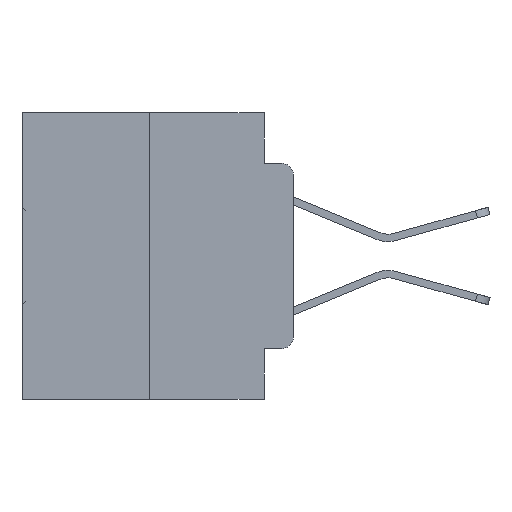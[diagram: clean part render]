
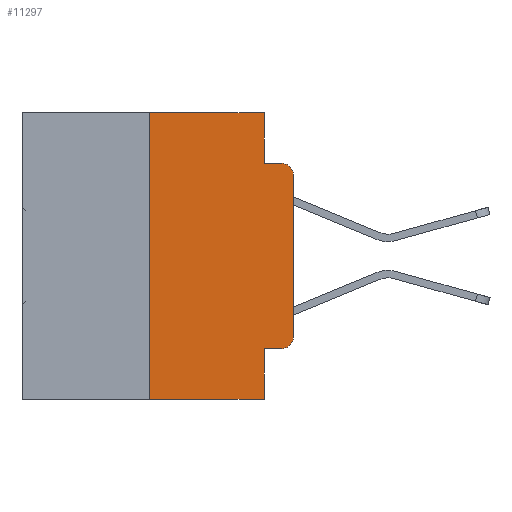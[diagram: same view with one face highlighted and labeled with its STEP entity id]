
A CAD part, left-side view. The second image highlights one B-rep face of the part: STEP entity #11297.
In plain terms, the highlighted planar face has unit normal (-1, 0, 0).
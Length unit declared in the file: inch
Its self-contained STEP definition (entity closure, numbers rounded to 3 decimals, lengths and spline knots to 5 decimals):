
#302 = DIRECTION ( 'NONE',  ( -1., 0., 0. ) ) ;
#361 = PLANE ( 'NONE',  #14105 ) ;
#1832 = EDGE_CURVE ( 'NONE', #31508, #29233, #28440, .T. ) ;
#3034 = VECTOR ( 'NONE', #4120, 39.37008 ) ;
#3745 = VECTOR ( 'NONE', #17222, 39.37008 ) ;
#3952 = DIRECTION ( 'NONE',  ( 0., -1., 0. ) ) ;
#4120 = DIRECTION ( 'NONE',  ( 0., 0., 1. ) ) ;
#5749 = ORIENTED_EDGE ( 'NONE', *, *, #12682, .T. ) ;
#5915 = DIRECTION ( 'NONE',  ( 0., 0., -1. ) ) ;
#6201 = LINE ( 'NONE', #6264, #7006 ) ;
#6264 = CARTESIAN_POINT ( 'NONE',  ( 0., 0.473, -0.5 ) ) ;
#7006 = VECTOR ( 'NONE', #24148, 39.37008 ) ;
#7079 = EDGE_CURVE ( 'NONE', #20912, #33186, #18273, .T. ) ;
#7255 = EDGE_LOOP ( 'NONE', ( #5749, #28667, #17162, #28207, #28958, #24762, #18702, #12947, #8277, #7651 ) ) ;
#7651 = ORIENTED_EDGE ( 'NONE', *, *, #7079, .T. ) ;
#7971 = LINE ( 'NONE', #11156, #21092 ) ;
#8277 = ORIENTED_EDGE ( 'NONE', *, *, #10899, .T. ) ;
#9403 = DIRECTION ( 'NONE',  ( 0., 0., -1. ) ) ;
#9429 = VECTOR ( 'NONE', #13624, 39.37008 ) ;
#9507 = CARTESIAN_POINT ( 'NONE',  ( 0., 0.02, -0.3915 ) ) ;
#10441 = CARTESIAN_POINT ( 'NONE',  ( 0., 0.051, 0. ) ) ;
#10899 = EDGE_CURVE ( 'NONE', #14200, #20912, #20010, .T. ) ;
#11002 = VERTEX_POINT ( 'NONE', #27409 ) ;
#11156 = CARTESIAN_POINT ( 'NONE',  ( 0., 0., 0. ) ) ;
#11297 = ADVANCED_FACE ( 'NONE', ( #21189 ), #361, .F. ) ;
#11696 = CARTESIAN_POINT ( 'NONE',  ( 0., 0.473, 0. ) ) ;
#12386 = VERTEX_POINT ( 'NONE', #24141 ) ;
#12682 = EDGE_CURVE ( 'NONE', #33186, #31508, #7971, .T. ) ;
#12947 = ORIENTED_EDGE ( 'NONE', *, *, #17543, .F. ) ;
#13279 = CARTESIAN_POINT ( 'NONE',  ( 0., 0.02, -0.1085 ) ) ;
#13501 = DIRECTION ( 'NONE',  ( 0., -1., 0. ) ) ;
#13624 = DIRECTION ( 'NONE',  ( 0., 0., -1. ) ) ;
#13856 = CARTESIAN_POINT ( 'NONE',  ( 0., 0., -0.1085 ) ) ;
#14105 = AXIS2_PLACEMENT_3D ( 'NONE', #24378, #16372, #5915 ) ;
#14200 = VERTEX_POINT ( 'NONE', #19577 ) ;
#14707 = EDGE_CURVE ( 'NONE', #12386, #29233, #19515, .T. ) ;
#16372 = DIRECTION ( 'NONE',  ( 1., 0., 0. ) ) ;
#16725 = EDGE_CURVE ( 'NONE', #23907, #30008, #27983, .T. ) ;
#17162 = ORIENTED_EDGE ( 'NONE', *, *, #14707, .F. ) ;
#17222 = DIRECTION ( 'NONE',  ( 0., -1., 0. ) ) ;
#17543 = EDGE_CURVE ( 'NONE', #14200, #18898, #30412, .T. ) ;
#18273 = CIRCLE ( 'NONE', #23080, 0.02 ) ;
#18702 = ORIENTED_EDGE ( 'NONE', *, *, #27818, .T. ) ;
#18712 = DIRECTION ( 'NONE',  ( 0., 0., -1. ) ) ;
#18898 = VERTEX_POINT ( 'NONE', #22165 ) ;
#18912 = DIRECTION ( 'NONE',  ( 0., 0., 1. ) ) ;
#19515 = LINE ( 'NONE', #32539, #25696 ) ;
#19577 = CARTESIAN_POINT ( 'NONE',  ( 0., 0.051, -0.4115 ) ) ;
#19688 = DIRECTION ( 'NONE',  ( 0., 0., -1. ) ) ;
#20010 = LINE ( 'NONE', #32227, #22914 ) ;
#20912 = VERTEX_POINT ( 'NONE', #33332 ) ;
#20940 = AXIS2_PLACEMENT_3D ( 'NONE', #13279, #302, #18712 ) ;
#21092 = VECTOR ( 'NONE', #18912, 39.37008 ) ;
#21101 = LINE ( 'NONE', #29957, #3034 ) ;
#21189 = FACE_OUTER_BOUND ( 'NONE', #7255, .T. ) ;
#21349 = LINE ( 'NONE', #10441, #9429 ) ;
#21358 = EDGE_CURVE ( 'NONE', #11002, #23907, #21101, .T. ) ;
#22165 = CARTESIAN_POINT ( 'NONE',  ( 0., 0.051, -0.5 ) ) ;
#22914 = VECTOR ( 'NONE', #13501, 39.37008 ) ;
#23080 = AXIS2_PLACEMENT_3D ( 'NONE', #9507, #30433, #9403 ) ;
#23406 = VECTOR ( 'NONE', #19688, 39.37008 ) ;
#23907 = VERTEX_POINT ( 'NONE', #26895 ) ;
#24141 = CARTESIAN_POINT ( 'NONE',  ( 0., 0.051, -0.0885 ) ) ;
#24148 = DIRECTION ( 'NONE',  ( 0., -1., 0. ) ) ;
#24378 = CARTESIAN_POINT ( 'NONE',  ( 0., 0.473, 0. ) ) ;
#24402 = EDGE_CURVE ( 'NONE', #30008, #12386, #21349, .T. ) ;
#24762 = ORIENTED_EDGE ( 'NONE', *, *, #21358, .F. ) ;
#25696 = VECTOR ( 'NONE', #3952, 39.37008 ) ;
#26895 = CARTESIAN_POINT ( 'NONE',  ( 0., 0.25, 0. ) ) ;
#27409 = CARTESIAN_POINT ( 'NONE',  ( 0., 0.25, -0.5 ) ) ;
#27818 = EDGE_CURVE ( 'NONE', #11002, #18898, #6201, .T. ) ;
#27983 = LINE ( 'NONE', #11696, #3745 ) ;
#28150 = CARTESIAN_POINT ( 'NONE',  ( 0., 0.051, 0. ) ) ;
#28207 = ORIENTED_EDGE ( 'NONE', *, *, #24402, .F. ) ;
#28440 = CIRCLE ( 'NONE', #20940, 0.02 ) ;
#28667 = ORIENTED_EDGE ( 'NONE', *, *, #1832, .T. ) ;
#28958 = ORIENTED_EDGE ( 'NONE', *, *, #16725, .F. ) ;
#29233 = VERTEX_POINT ( 'NONE', #30620 ) ;
#29957 = CARTESIAN_POINT ( 'NONE',  ( 0., 0.25, 0. ) ) ;
#30008 = VERTEX_POINT ( 'NONE', #28150 ) ;
#30412 = LINE ( 'NONE', #32796, #23406 ) ;
#30433 = DIRECTION ( 'NONE',  ( -1., 0., 0. ) ) ;
#30620 = CARTESIAN_POINT ( 'NONE',  ( 0., 0.02, -0.0885 ) ) ;
#31476 = CARTESIAN_POINT ( 'NONE',  ( 0., 0., -0.3915 ) ) ;
#31508 = VERTEX_POINT ( 'NONE', #13856 ) ;
#32227 = CARTESIAN_POINT ( 'NONE',  ( 0., 0.051, -0.4115 ) ) ;
#32539 = CARTESIAN_POINT ( 'NONE',  ( 0., 0.051, -0.0885 ) ) ;
#32796 = CARTESIAN_POINT ( 'NONE',  ( 0., 0.051, 0. ) ) ;
#33186 = VERTEX_POINT ( 'NONE', #31476 ) ;
#33332 = CARTESIAN_POINT ( 'NONE',  ( 0., 0.02, -0.4115 ) ) ;
